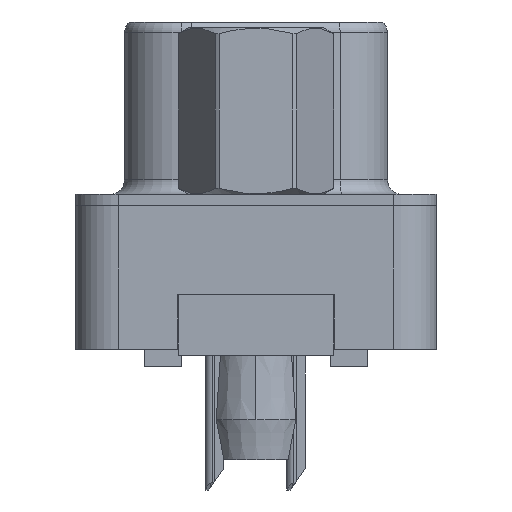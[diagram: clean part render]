
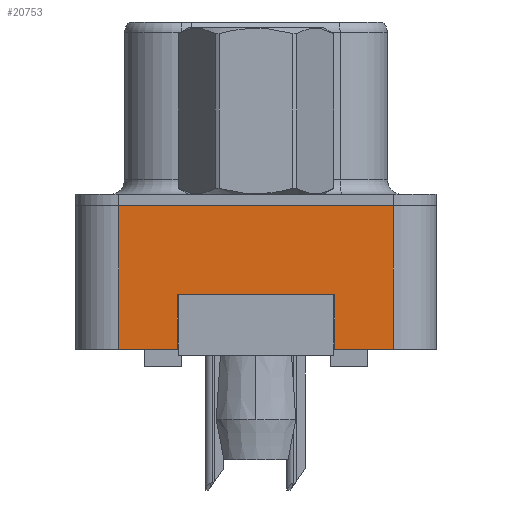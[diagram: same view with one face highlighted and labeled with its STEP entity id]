
A CAD part, left-side view. The second image highlights one B-rep face of the part: STEP entity #20753.
In plain terms, the highlighted planar face has unit normal (-1, 0, 0).
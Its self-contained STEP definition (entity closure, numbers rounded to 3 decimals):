
#1559 = LINE ( 'NONE', #11931, #4825 ) ;
#2397 = VERTEX_POINT ( 'NONE', #25080 ) ;
#2661 = EDGE_CURVE ( 'NONE', #13787, #10007, #11090, .T. ) ;
#2675 = CARTESIAN_POINT ( 'NONE',  ( -2.91, -4.775, -5. ) ) ;
#2887 = VECTOR ( 'NONE', #32317, 1000. ) ;
#3918 = FACE_OUTER_BOUND ( 'NONE', #4815, .T. ) ;
#4250 = ORIENTED_EDGE ( 'NONE', *, *, #2661, .F. ) ;
#4815 = EDGE_LOOP ( 'NONE', ( #7413, #32443, #24580, #5498, #4250, #15786, #15182, #24085 ) ) ;
#4825 = VECTOR ( 'NONE', #32718, 1000. ) ;
#5322 = VERTEX_POINT ( 'NONE', #13245 ) ;
#5498 = ORIENTED_EDGE ( 'NONE', *, *, #15161, .F. ) ;
#5603 = LINE ( 'NONE', #8165, #18717 ) ;
#6297 = DIRECTION ( 'NONE',  ( -1., 0., 0. ) ) ;
#6305 = EDGE_CURVE ( 'NONE', #5322, #9504, #26490, .T. ) ;
#6605 = VERTEX_POINT ( 'NONE', #9762 ) ;
#7139 = CARTESIAN_POINT ( 'NONE',  ( -2.91, 2.75, -5. ) ) ;
#7241 = LINE ( 'NONE', #17610, #13235 ) ;
#7413 = ORIENTED_EDGE ( 'NONE', *, *, #29895, .T. ) ;
#8165 = CARTESIAN_POINT ( 'NONE',  ( -2.91, -4.775, -5. ) ) ;
#8389 = LINE ( 'NONE', #26769, #24640 ) ;
#9504 = VERTEX_POINT ( 'NONE', #32768 ) ;
#9762 = CARTESIAN_POINT ( 'NONE',  ( -2.91, -4.775, 0. ) ) ;
#9862 = VECTOR ( 'NONE', #10674, 1000. ) ;
#10007 = VERTEX_POINT ( 'NONE', #10047 ) ;
#10047 = CARTESIAN_POINT ( 'NONE',  ( -2.91, 4.775, 0. ) ) ;
#10674 = DIRECTION ( 'NONE',  ( 0., 0., 1. ) ) ;
#11090 = LINE ( 'NONE', #13959, #15005 ) ;
#11264 = DIRECTION ( 'NONE',  ( 0., -1., 0. ) ) ;
#11406 = PLANE ( 'NONE',  #21243 ) ;
#11500 = EDGE_CURVE ( 'NONE', #2397, #6605, #30948, .T. ) ;
#11931 = CARTESIAN_POINT ( 'NONE',  ( -2.91, -2.75, -3.1 ) ) ;
#12082 = VERTEX_POINT ( 'NONE', #20201 ) ;
#13007 = CARTESIAN_POINT ( 'NONE',  ( -2.91, 4.775, -5. ) ) ;
#13235 = VECTOR ( 'NONE', #28014, 1000. ) ;
#13245 = CARTESIAN_POINT ( 'NONE',  ( -2.91, -2.75, -3.1 ) ) ;
#13745 = EDGE_CURVE ( 'NONE', #13787, #32856, #7241, .T. ) ;
#13787 = VERTEX_POINT ( 'NONE', #13007 ) ;
#13959 = CARTESIAN_POINT ( 'NONE',  ( -2.91, 4.775, -5. ) ) ;
#15005 = VECTOR ( 'NONE', #18583, 1000. ) ;
#15161 = EDGE_CURVE ( 'NONE', #10007, #6605, #8389, .T. ) ;
#15182 = ORIENTED_EDGE ( 'NONE', *, *, #25045, .F. ) ;
#15786 = ORIENTED_EDGE ( 'NONE', *, *, #13745, .T. ) ;
#15971 = DIRECTION ( 'NONE',  ( 0., -1., 0. ) ) ;
#16466 = CARTESIAN_POINT ( 'NONE',  ( -2.91, 2.75, -3.1 ) ) ;
#16648 = EDGE_CURVE ( 'NONE', #12082, #2397, #5603, .T. ) ;
#16675 = DIRECTION ( 'NONE',  ( 0., 0., 1. ) ) ;
#17610 = CARTESIAN_POINT ( 'NONE',  ( -2.91, -4.775, -5. ) ) ;
#18583 = DIRECTION ( 'NONE',  ( 0., 0., 1. ) ) ;
#18717 = VECTOR ( 'NONE', #15971, 1000. ) ;
#19231 = CARTESIAN_POINT ( 'NONE',  ( -2.91, -4.775, -5. ) ) ;
#20201 = CARTESIAN_POINT ( 'NONE',  ( -2.91, -2.75, -5. ) ) ;
#20753 = ADVANCED_FACE ( 'NONE', ( #3918 ), #11406, .T. ) ;
#21243 = AXIS2_PLACEMENT_3D ( 'NONE', #19231, #6297, #16675 ) ;
#21752 = LINE ( 'NONE', #16466, #2887 ) ;
#23928 = DIRECTION ( 'NONE',  ( 0., 1., 0. ) ) ;
#24085 = ORIENTED_EDGE ( 'NONE', *, *, #6305, .F. ) ;
#24580 = ORIENTED_EDGE ( 'NONE', *, *, #11500, .T. ) ;
#24640 = VECTOR ( 'NONE', #11264, 1000. ) ;
#25045 = EDGE_CURVE ( 'NONE', #9504, #32856, #21752, .T. ) ;
#25080 = CARTESIAN_POINT ( 'NONE',  ( -2.91, -4.775, -5. ) ) ;
#26490 = LINE ( 'NONE', #29208, #28112 ) ;
#26769 = CARTESIAN_POINT ( 'NONE',  ( -2.91, -4.775, 0. ) ) ;
#28014 = DIRECTION ( 'NONE',  ( 0., -1., 0. ) ) ;
#28112 = VECTOR ( 'NONE', #23928, 1000. ) ;
#29208 = CARTESIAN_POINT ( 'NONE',  ( -2.91, 2.75, -3.1 ) ) ;
#29895 = EDGE_CURVE ( 'NONE', #5322, #12082, #1559, .T. ) ;
#30948 = LINE ( 'NONE', #2675, #9862 ) ;
#32317 = DIRECTION ( 'NONE',  ( 0., 0., -1. ) ) ;
#32443 = ORIENTED_EDGE ( 'NONE', *, *, #16648, .T. ) ;
#32718 = DIRECTION ( 'NONE',  ( 0., 0., -1. ) ) ;
#32768 = CARTESIAN_POINT ( 'NONE',  ( -2.91, 2.75, -3.1 ) ) ;
#32856 = VERTEX_POINT ( 'NONE', #7139 ) ;
